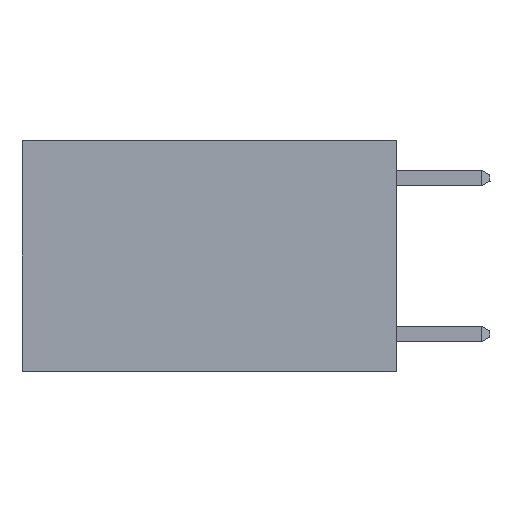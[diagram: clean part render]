
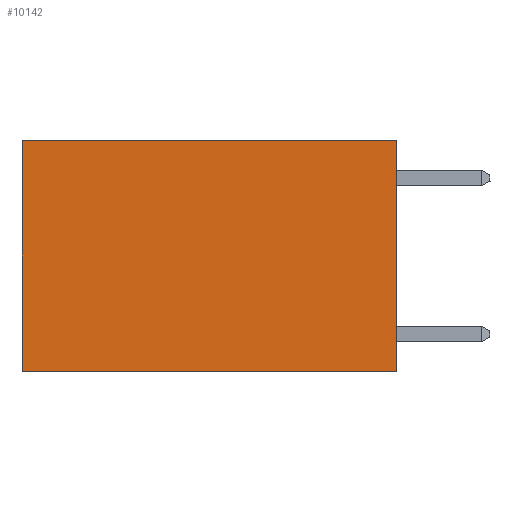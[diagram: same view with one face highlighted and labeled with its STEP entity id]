
A CAD part, left-side view. The second image highlights one B-rep face of the part: STEP entity #10142.
In plain terms, the highlighted planar face has unit normal (-1, 0, 0).
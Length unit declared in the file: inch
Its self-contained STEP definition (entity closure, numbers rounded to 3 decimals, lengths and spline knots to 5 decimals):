
#664 = DIRECTION ( 'NONE',  ( 0., 0., -1. ) ) ;
#891 = VERTEX_POINT ( 'NONE', #13514 ) ;
#1274 = ORIENTED_EDGE ( 'NONE', *, *, #5376, .F. ) ;
#1401 = FACE_OUTER_BOUND ( 'NONE', #13993, .T. ) ;
#1764 = ORIENTED_EDGE ( 'NONE', *, *, #10809, .F. ) ;
#2854 = VECTOR ( 'NONE', #15231, 39.37008 ) ;
#3068 = LINE ( 'NONE', #3678, #7094 ) ;
#3678 = CARTESIAN_POINT ( 'NONE',  ( 0.2625, 0., 0. ) ) ;
#3928 = CARTESIAN_POINT ( 'NONE',  ( 0.2625, 0.6, -0.37 ) ) ;
#4056 = AXIS2_PLACEMENT_3D ( 'NONE', #4583, #14021, #5949 ) ;
#4082 = VECTOR ( 'NONE', #14226, 39.37008 ) ;
#4583 = CARTESIAN_POINT ( 'NONE',  ( 0.2625, 0., 0. ) ) ;
#4935 = VERTEX_POINT ( 'NONE', #8154 ) ;
#5376 = EDGE_CURVE ( 'NONE', #4935, #9342, #14849, .T. ) ;
#5508 = ORIENTED_EDGE ( 'NONE', *, *, #6529, .T. ) ;
#5949 = DIRECTION ( 'NONE',  ( 0., 0., -1. ) ) ;
#6367 = DIRECTION ( 'NONE',  ( 0., 1., 0. ) ) ;
#6529 = EDGE_CURVE ( 'NONE', #7609, #891, #14818, .T. ) ;
#7094 = VECTOR ( 'NONE', #664, 39.37008 ) ;
#7609 = VERTEX_POINT ( 'NONE', #14889 ) ;
#8154 = CARTESIAN_POINT ( 'NONE',  ( 0.2625, 0., -0.37 ) ) ;
#8597 = PLANE ( 'NONE',  #4056 ) ;
#9342 = VERTEX_POINT ( 'NONE', #3928 ) ;
#10058 = EDGE_CURVE ( 'NONE', #891, #9342, #13637, .T. ) ;
#10142 = ADVANCED_FACE ( 'NONE', ( #1401 ), #8597, .F. ) ;
#10809 = EDGE_CURVE ( 'NONE', #7609, #4935, #3068, .T. ) ;
#11624 = CARTESIAN_POINT ( 'NONE',  ( 0.2625, 0., -0.37 ) ) ;
#13134 = CARTESIAN_POINT ( 'NONE',  ( 0.2625, 0., 0. ) ) ;
#13514 = CARTESIAN_POINT ( 'NONE',  ( 0.2625, 0.6, 0. ) ) ;
#13637 = LINE ( 'NONE', #13856, #2854 ) ;
#13856 = CARTESIAN_POINT ( 'NONE',  ( 0.2625, 0.6, 0. ) ) ;
#13993 = EDGE_LOOP ( 'NONE', ( #15424, #1274, #1764, #5508 ) ) ;
#14021 = DIRECTION ( 'NONE',  ( 1., 0., 0. ) ) ;
#14226 = DIRECTION ( 'NONE',  ( 0., 1., 0. ) ) ;
#14390 = VECTOR ( 'NONE', #6367, 39.37008 ) ;
#14818 = LINE ( 'NONE', #13134, #14390 ) ;
#14849 = LINE ( 'NONE', #11624, #4082 ) ;
#14889 = CARTESIAN_POINT ( 'NONE',  ( 0.2625, 0., 0. ) ) ;
#15231 = DIRECTION ( 'NONE',  ( 0., 0., -1. ) ) ;
#15424 = ORIENTED_EDGE ( 'NONE', *, *, #10058, .T. ) ;
